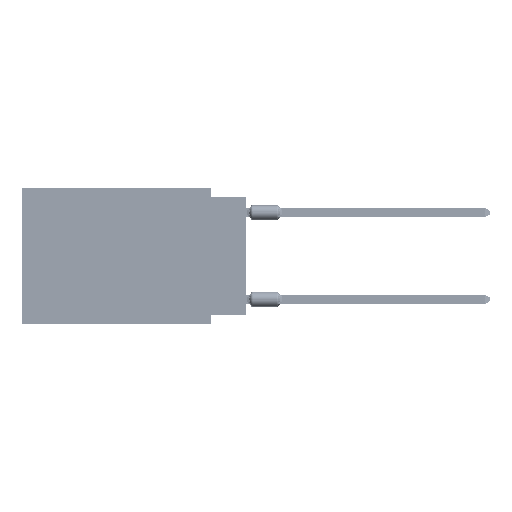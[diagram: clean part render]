
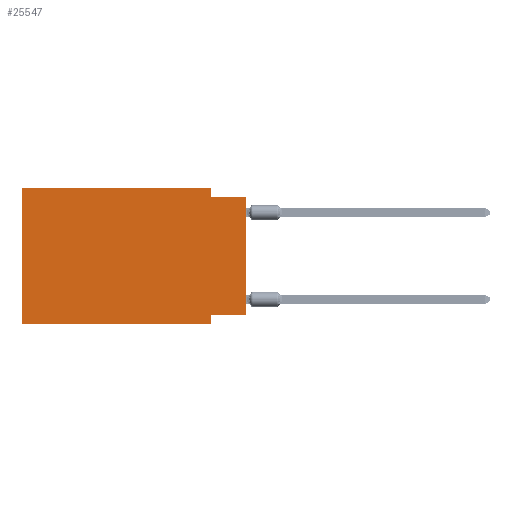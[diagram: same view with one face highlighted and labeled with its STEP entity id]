
A CAD part, left-side view. The second image highlights one B-rep face of the part: STEP entity #25547.
In plain terms, the highlighted planar face has unit normal (-1, 0, 0).
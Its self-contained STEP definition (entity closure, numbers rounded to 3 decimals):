
#588 = VERTEX_POINT ( 'NONE', #14874 ) ;
#1895 = CARTESIAN_POINT ( 'NONE',  ( 0., 16.383, -9.906 ) ) ;
#2600 = LINE ( 'NONE', #8400, #17565 ) ;
#2626 = LINE ( 'NONE', #46960, #70658 ) ;
#2950 = DIRECTION ( 'NONE',  ( 0., 1., 0. ) ) ;
#3027 = LINE ( 'NONE', #7048, #53107 ) ;
#3287 = VERTEX_POINT ( 'NONE', #57483 ) ;
#3813 = ORIENTED_EDGE ( 'NONE', *, *, #34030, .F. ) ;
#3951 = LINE ( 'NONE', #19580, #30688 ) ;
#4615 = EDGE_CURVE ( 'NONE', #65065, #13598, #2626, .T. ) ;
#5168 = VECTOR ( 'NONE', #32505, 1000. ) ;
#7048 = CARTESIAN_POINT ( 'NONE',  ( 0., 2.54, 0. ) ) ;
#8400 = CARTESIAN_POINT ( 'NONE',  ( 0., 0., -9.271 ) ) ;
#9215 = EDGE_CURVE ( 'NONE', #65065, #3287, #62592, .T. ) ;
#11151 = LINE ( 'NONE', #70786, #52149 ) ;
#11186 = VERTEX_POINT ( 'NONE', #34027 ) ;
#13573 = DIRECTION ( 'NONE',  ( 0., 0., -1. ) ) ;
#13598 = VERTEX_POINT ( 'NONE', #16329 ) ;
#14874 = CARTESIAN_POINT ( 'NONE',  ( 0., 0., -0.635 ) ) ;
#14955 = CARTESIAN_POINT ( 'NONE',  ( 0., 2.54, -9.271 ) ) ;
#16321 = EDGE_CURVE ( 'NONE', #20194, #3287, #3951, .T. ) ;
#16329 = CARTESIAN_POINT ( 'NONE',  ( 0., 16.383, 0. ) ) ;
#17565 = VECTOR ( 'NONE', #2950, 1000. ) ;
#17816 = LINE ( 'NONE', #57074, #65527 ) ;
#19580 = CARTESIAN_POINT ( 'NONE',  ( 0., 2.54, -9.906 ) ) ;
#20194 = VERTEX_POINT ( 'NONE', #14955 ) ;
#21301 = VERTEX_POINT ( 'NONE', #28897 ) ;
#23627 = ORIENTED_EDGE ( 'NONE', *, *, #64094, .F. ) ;
#25547 = ADVANCED_FACE ( 'NONE', ( #71804 ), #60521, .F. ) ;
#28252 = EDGE_CURVE ( 'NONE', #13598, #21301, #37952, .T. ) ;
#28897 = CARTESIAN_POINT ( 'NONE',  ( 0., 2.54, 0. ) ) ;
#29281 = CARTESIAN_POINT ( 'NONE',  ( 0., 0., -9.271 ) ) ;
#29832 = ORIENTED_EDGE ( 'NONE', *, *, #16321, .F. ) ;
#30229 = DIRECTION ( 'NONE',  ( 0., -1., 0. ) ) ;
#30688 = VECTOR ( 'NONE', #47204, 1000. ) ;
#32505 = DIRECTION ( 'NONE',  ( 0., -1., 0. ) ) ;
#34027 = CARTESIAN_POINT ( 'NONE',  ( 0., 2.54, -0.635 ) ) ;
#34030 = EDGE_CURVE ( 'NONE', #21301, #11186, #3027, .T. ) ;
#35165 = EDGE_LOOP ( 'NONE', ( #63648, #42058, #3813, #50445, #52207, #67538, #29832, #23627 ) ) ;
#37952 = LINE ( 'NONE', #55769, #5168 ) ;
#39178 = EDGE_CURVE ( 'NONE', #11186, #588, #11151, .T. ) ;
#42058 = ORIENTED_EDGE ( 'NONE', *, *, #39178, .F. ) ;
#43826 = DIRECTION ( 'NONE',  ( 0., 0., -1. ) ) ;
#46960 = CARTESIAN_POINT ( 'NONE',  ( 0., 16.383, 0. ) ) ;
#47204 = DIRECTION ( 'NONE',  ( 0., 0., -1. ) ) ;
#47350 = EDGE_CURVE ( 'NONE', #48953, #588, #17816, .T. ) ;
#48953 = VERTEX_POINT ( 'NONE', #29281 ) ;
#49265 = CARTESIAN_POINT ( 'NONE',  ( 0., 16.383, 0. ) ) ;
#50445 = ORIENTED_EDGE ( 'NONE', *, *, #28252, .F. ) ;
#52149 = VECTOR ( 'NONE', #55134, 1000. ) ;
#52207 = ORIENTED_EDGE ( 'NONE', *, *, #4615, .F. ) ;
#52491 = AXIS2_PLACEMENT_3D ( 'NONE', #49265, #70109, #43826 ) ;
#52570 = CARTESIAN_POINT ( 'NONE',  ( 0., 16.383, -9.906 ) ) ;
#53107 = VECTOR ( 'NONE', #13573, 1000. ) ;
#55134 = DIRECTION ( 'NONE',  ( 0., -1., 0. ) ) ;
#55769 = CARTESIAN_POINT ( 'NONE',  ( 0., 16.383, 0. ) ) ;
#56008 = DIRECTION ( 'NONE',  ( 0., 0., 1. ) ) ;
#57074 = CARTESIAN_POINT ( 'NONE',  ( 0., 0., 0. ) ) ;
#57483 = CARTESIAN_POINT ( 'NONE',  ( 0., 2.54, -9.906 ) ) ;
#57859 = DIRECTION ( 'NONE',  ( 0., 0., 1. ) ) ;
#60521 = PLANE ( 'NONE',  #52491 ) ;
#61358 = VECTOR ( 'NONE', #30229, 1000. ) ;
#62592 = LINE ( 'NONE', #1895, #61358 ) ;
#63648 = ORIENTED_EDGE ( 'NONE', *, *, #47350, .T. ) ;
#64094 = EDGE_CURVE ( 'NONE', #48953, #20194, #2600, .T. ) ;
#65065 = VERTEX_POINT ( 'NONE', #52570 ) ;
#65527 = VECTOR ( 'NONE', #56008, 1000. ) ;
#67538 = ORIENTED_EDGE ( 'NONE', *, *, #9215, .T. ) ;
#70109 = DIRECTION ( 'NONE',  ( 1., 0., 0. ) ) ;
#70658 = VECTOR ( 'NONE', #57859, 1000. ) ;
#70786 = CARTESIAN_POINT ( 'NONE',  ( 0., 0., -0.635 ) ) ;
#71804 = FACE_OUTER_BOUND ( 'NONE', #35165, .T. ) ;
